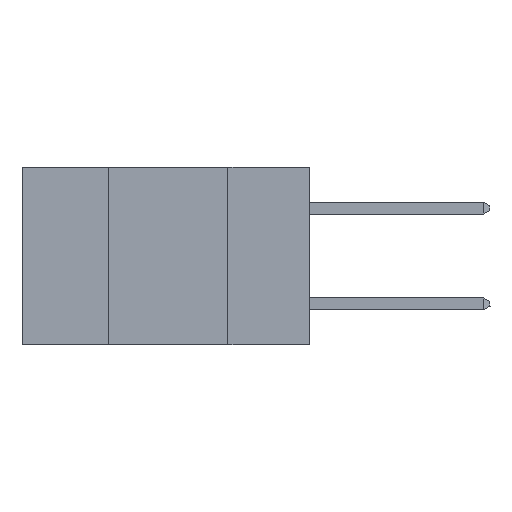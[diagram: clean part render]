
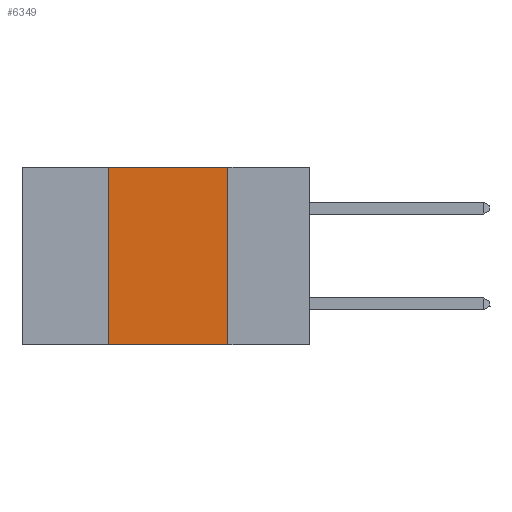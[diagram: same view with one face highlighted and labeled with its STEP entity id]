
A CAD part, left-side view. The second image highlights one B-rep face of the part: STEP entity #6349.
In plain terms, the highlighted planar face has unit normal (-1, 0, 0).
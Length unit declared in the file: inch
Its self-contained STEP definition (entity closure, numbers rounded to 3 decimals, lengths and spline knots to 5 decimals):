
#389 = VERTEX_POINT ( 'NONE', #8599 ) ;
#872 = EDGE_CURVE ( 'NONE', #3031, #6271, #13402, .T. ) ;
#1240 = PLANE ( 'NONE',  #16797 ) ;
#1244 = LINE ( 'NONE', #5358, #12131 ) ;
#1312 = CARTESIAN_POINT ( 'NONE',  ( 0., 0.17, 0. ) ) ;
#2750 = CARTESIAN_POINT ( 'NONE',  ( 0., 0.17, -0.37 ) ) ;
#2873 = DIRECTION ( 'NONE',  ( 0., -1., 0. ) ) ;
#3031 = VERTEX_POINT ( 'NONE', #7962 ) ;
#3320 = ORIENTED_EDGE ( 'NONE', *, *, #4009, .T. ) ;
#3818 = VECTOR ( 'NONE', #8169, 39.37008 ) ;
#4009 = EDGE_CURVE ( 'NONE', #18006, #6271, #8008, .T. ) ;
#4906 = VECTOR ( 'NONE', #7814, 39.37008 ) ;
#5358 = CARTESIAN_POINT ( 'NONE',  ( 0., 0.6, 0. ) ) ;
#5391 = CARTESIAN_POINT ( 'NONE',  ( 0., 0.6, -0.37 ) ) ;
#5478 = ORIENTED_EDGE ( 'NONE', *, *, #6782, .F. ) ;
#5544 = ORIENTED_EDGE ( 'NONE', *, *, #6151, .F. ) ;
#5785 = VECTOR ( 'NONE', #8074, 39.37008 ) ;
#6151 = EDGE_CURVE ( 'NONE', #389, #3031, #1244, .T. ) ;
#6271 = VERTEX_POINT ( 'NONE', #2750 ) ;
#6349 = ADVANCED_FACE ( 'NONE', ( #17161 ), #1240, .F. ) ;
#6782 = EDGE_CURVE ( 'NONE', #18006, #389, #8601, .T. ) ;
#7814 = DIRECTION ( 'NONE',  ( 0., 0., 1. ) ) ;
#7962 = CARTESIAN_POINT ( 'NONE',  ( 0., 0.17, 0. ) ) ;
#7990 = ORIENTED_EDGE ( 'NONE', *, *, #872, .F. ) ;
#8008 = LINE ( 'NONE', #5391, #5785 ) ;
#8074 = DIRECTION ( 'NONE',  ( 0., -1., 0. ) ) ;
#8169 = DIRECTION ( 'NONE',  ( 0., 0., -1. ) ) ;
#8599 = CARTESIAN_POINT ( 'NONE',  ( 0., 0.42, 0. ) ) ;
#8601 = LINE ( 'NONE', #8911, #4906 ) ;
#8911 = CARTESIAN_POINT ( 'NONE',  ( 0., 0.42, 0. ) ) ;
#12131 = VECTOR ( 'NONE', #2873, 39.37008 ) ;
#12366 = DIRECTION ( 'NONE',  ( 0., 0., -1. ) ) ;
#12484 = DIRECTION ( 'NONE',  ( 1., 0., 0. ) ) ;
#13402 = LINE ( 'NONE', #1312, #3818 ) ;
#13523 = EDGE_LOOP ( 'NONE', ( #7990, #5544, #5478, #3320 ) ) ;
#13698 = CARTESIAN_POINT ( 'NONE',  ( 0., 0.6, 0. ) ) ;
#14533 = CARTESIAN_POINT ( 'NONE',  ( 0., 0.42, -0.37 ) ) ;
#16797 = AXIS2_PLACEMENT_3D ( 'NONE', #13698, #12484, #12366 ) ;
#17161 = FACE_OUTER_BOUND ( 'NONE', #13523, .T. ) ;
#18006 = VERTEX_POINT ( 'NONE', #14533 ) ;
